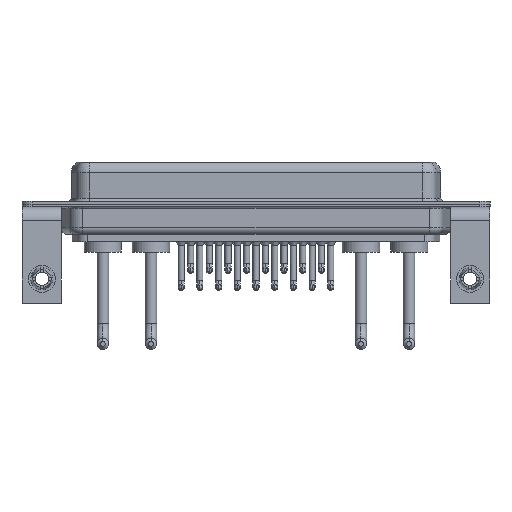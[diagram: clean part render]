
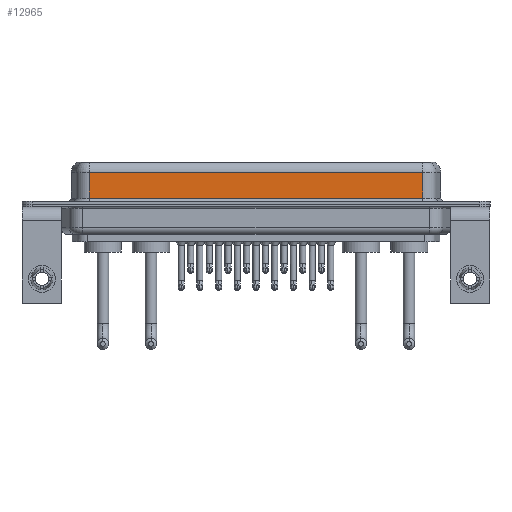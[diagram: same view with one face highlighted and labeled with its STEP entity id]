
A CAD part, front view. The second image highlights one B-rep face of the part: STEP entity #12965.
In plain terms, the highlighted planar face has unit normal (0, -1, 0).
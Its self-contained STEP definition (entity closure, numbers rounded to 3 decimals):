
#174 = VECTOR ( 'NONE', #15112, 1000. ) ;
#881 = AXIS2_PLACEMENT_3D ( 'NONE', #18597, #9206, #5736 ) ;
#885 = LINE ( 'NONE', #8567, #1905 ) ;
#1562 = VECTOR ( 'NONE', #7689, 1000. ) ;
#1905 = VECTOR ( 'NONE', #4505, 1000. ) ;
#2660 = CARTESIAN_POINT ( 'NONE',  ( 56.462, -3.95, 0.9 ) ) ;
#3507 = PLANE ( 'NONE',  #881 ) ;
#3520 = EDGE_CURVE ( 'NONE', #12274, #15250, #20916, .T. ) ;
#4505 = DIRECTION ( 'NONE',  ( 1., 0., 0. ) ) ;
#5459 = CARTESIAN_POINT ( 'NONE',  ( 7.038, -3.95, 6.4 ) ) ;
#5736 = DIRECTION ( 'NONE',  ( 0., 0., 1. ) ) ;
#5763 = ORIENTED_EDGE ( 'NONE', *, *, #6692, .T. ) ;
#6692 = EDGE_CURVE ( 'NONE', #8242, #21308, #885, .T. ) ;
#7139 = CARTESIAN_POINT ( 'NONE',  ( 56.462, -3.95, 4.65 ) ) ;
#7689 = DIRECTION ( 'NONE',  ( -1., 0., 0. ) ) ;
#8201 = CARTESIAN_POINT ( 'NONE',  ( 56.462, -3.95, 6.4 ) ) ;
#8242 = VERTEX_POINT ( 'NONE', #24209 ) ;
#8268 = ORIENTED_EDGE ( 'NONE', *, *, #3520, .T. ) ;
#8567 = CARTESIAN_POINT ( 'NONE',  ( 56.462, -3.95, 0.9 ) ) ;
#9206 = DIRECTION ( 'NONE',  ( 0., 1., 0. ) ) ;
#9435 = CARTESIAN_POINT ( 'NONE',  ( 56.462, -3.95, 4.65 ) ) ;
#9637 = ORIENTED_EDGE ( 'NONE', *, *, #19640, .F. ) ;
#12274 = VERTEX_POINT ( 'NONE', #7139 ) ;
#12359 = VECTOR ( 'NONE', #17720, 1000. ) ;
#12965 = ADVANCED_FACE ( 'NONE', ( #20454 ), #3507, .F. ) ;
#12986 = EDGE_LOOP ( 'NONE', ( #9637, #8268, #20294, #5763 ) ) ;
#14813 = CARTESIAN_POINT ( 'NONE',  ( 7.038, -3.95, 4.65 ) ) ;
#15112 = DIRECTION ( 'NONE',  ( 0., 0., -1. ) ) ;
#15250 = VERTEX_POINT ( 'NONE', #14813 ) ;
#17720 = DIRECTION ( 'NONE',  ( 0., 0., -1. ) ) ;
#18597 = CARTESIAN_POINT ( 'NONE',  ( 56.462, -3.95, 6.4 ) ) ;
#18804 = LINE ( 'NONE', #5459, #174 ) ;
#19640 = EDGE_CURVE ( 'NONE', #12274, #21308, #21295, .T. ) ;
#20294 = ORIENTED_EDGE ( 'NONE', *, *, #23479, .T. ) ;
#20454 = FACE_OUTER_BOUND ( 'NONE', #12986, .T. ) ;
#20916 = LINE ( 'NONE', #9435, #1562 ) ;
#21295 = LINE ( 'NONE', #8201, #12359 ) ;
#21308 = VERTEX_POINT ( 'NONE', #2660 ) ;
#23479 = EDGE_CURVE ( 'NONE', #15250, #8242, #18804, .T. ) ;
#24209 = CARTESIAN_POINT ( 'NONE',  ( 7.038, -3.95, 0.9 ) ) ;
